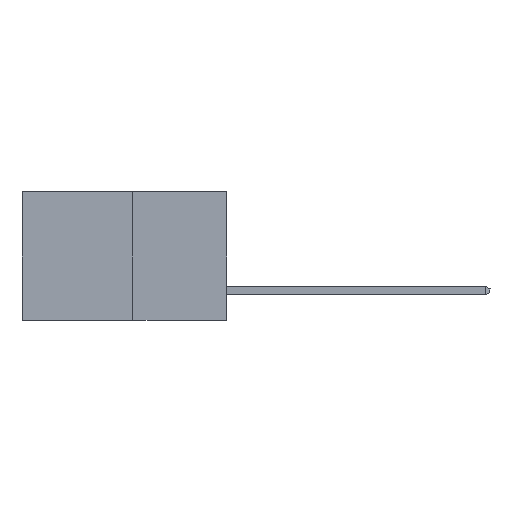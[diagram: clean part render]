
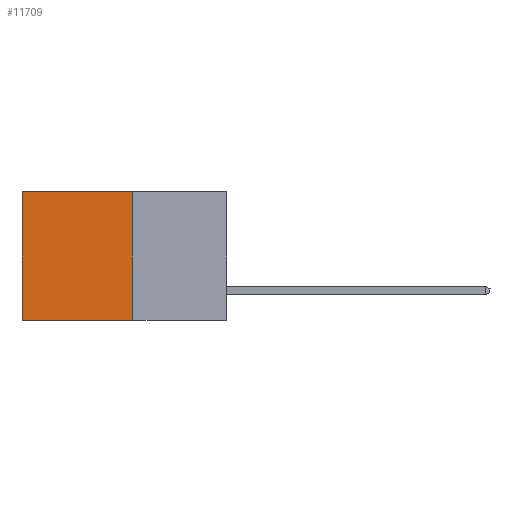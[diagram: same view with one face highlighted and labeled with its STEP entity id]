
A CAD part, left-side view. The second image highlights one B-rep face of the part: STEP entity #11709.
In plain terms, the highlighted planar face has unit normal (-1, 0, 0).
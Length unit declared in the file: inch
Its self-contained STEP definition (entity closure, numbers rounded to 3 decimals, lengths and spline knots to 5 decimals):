
#862 = CARTESIAN_POINT ( 'NONE',  ( 0.277, 0.27, -0.37 ) ) ;
#1999 = DIRECTION ( 'NONE',  ( 0., 1., 0. ) ) ;
#2284 = DIRECTION ( 'NONE',  ( 0., 0., -1. ) ) ;
#2934 = FACE_OUTER_BOUND ( 'NONE', #16683, .T. ) ;
#3264 = VERTEX_POINT ( 'NONE', #4985 ) ;
#4277 = EDGE_CURVE ( 'NONE', #15204, #15195, #7191, .T. ) ;
#4662 = LINE ( 'NONE', #13391, #11791 ) ;
#4985 = CARTESIAN_POINT ( 'NONE',  ( 0.277, 0.59, -0.37 ) ) ;
#5388 = CARTESIAN_POINT ( 'NONE',  ( 0.277, 0.27, -0.37 ) ) ;
#5554 = AXIS2_PLACEMENT_3D ( 'NONE', #862, #10816, #2284 ) ;
#5943 = CARTESIAN_POINT ( 'NONE',  ( 0.277, 0.59, 0. ) ) ;
#6058 = ORIENTED_EDGE ( 'NONE', *, *, #14443, .T. ) ;
#6534 = PLANE ( 'NONE',  #5554 ) ;
#6869 = DIRECTION ( 'NONE',  ( 0., 0., -1. ) ) ;
#6983 = ORIENTED_EDGE ( 'NONE', *, *, #11835, .F. ) ;
#7191 = LINE ( 'NONE', #16021, #13826 ) ;
#7341 = LINE ( 'NONE', #9973, #18098 ) ;
#8347 = LINE ( 'NONE', #5388, #15389 ) ;
#8849 = CARTESIAN_POINT ( 'NONE',  ( 0.277, 0.27, 0. ) ) ;
#9973 = CARTESIAN_POINT ( 'NONE',  ( 0.277, 0.59, -0.37 ) ) ;
#10816 = DIRECTION ( 'NONE',  ( 1., 0., 0. ) ) ;
#11709 = ADVANCED_FACE ( 'NONE', ( #2934 ), #6534, .F. ) ;
#11791 = VECTOR ( 'NONE', #1999, 39.37008 ) ;
#11835 = EDGE_CURVE ( 'NONE', #15204, #13050, #8347, .T. ) ;
#12202 = CARTESIAN_POINT ( 'NONE',  ( 0.277, 0.27, -0.37 ) ) ;
#12924 = EDGE_CURVE ( 'NONE', #13050, #3264, #4662, .T. ) ;
#13050 = VERTEX_POINT ( 'NONE', #12202 ) ;
#13391 = CARTESIAN_POINT ( 'NONE',  ( 0.277, 0.27, -0.37 ) ) ;
#13605 = ORIENTED_EDGE ( 'NONE', *, *, #12924, .F. ) ;
#13826 = VECTOR ( 'NONE', #15848, 39.37008 ) ;
#14443 = EDGE_CURVE ( 'NONE', #15195, #3264, #7341, .T. ) ;
#14939 = ORIENTED_EDGE ( 'NONE', *, *, #4277, .T. ) ;
#15195 = VERTEX_POINT ( 'NONE', #5943 ) ;
#15204 = VERTEX_POINT ( 'NONE', #8849 ) ;
#15389 = VECTOR ( 'NONE', #6869, 39.37008 ) ;
#15848 = DIRECTION ( 'NONE',  ( 0., 1., 0. ) ) ;
#16021 = CARTESIAN_POINT ( 'NONE',  ( 0.277, 0.27, 0. ) ) ;
#16683 = EDGE_LOOP ( 'NONE', ( #6058, #13605, #6983, #14939 ) ) ;
#16931 = DIRECTION ( 'NONE',  ( 0., 0., -1. ) ) ;
#18098 = VECTOR ( 'NONE', #16931, 39.37008 ) ;
